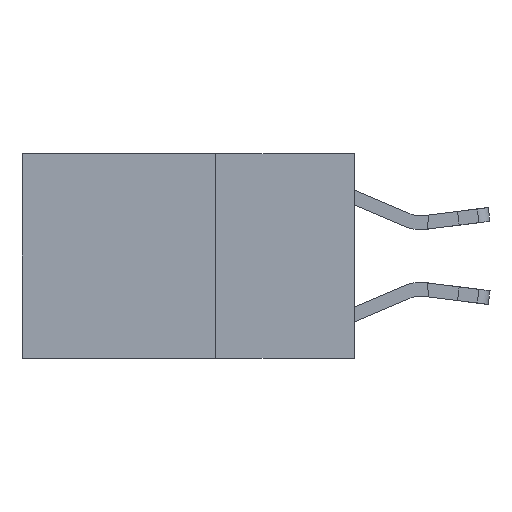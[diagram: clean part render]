
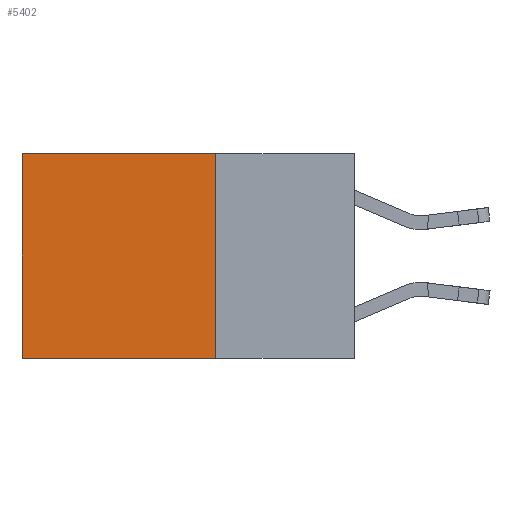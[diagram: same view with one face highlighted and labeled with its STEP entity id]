
A CAD part, left-side view. The second image highlights one B-rep face of the part: STEP entity #5402.
In plain terms, the highlighted planar face has unit normal (-1, 0, 0).
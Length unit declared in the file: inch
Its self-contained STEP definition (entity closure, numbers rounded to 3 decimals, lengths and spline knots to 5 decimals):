
#186 = VERTEX_POINT ( 'NONE', #7719 ) ;
#538 = FACE_OUTER_BOUND ( 'NONE', #6070, .T. ) ;
#646 = CARTESIAN_POINT ( 'NONE',  ( 0.2625, 0.25, -0.37 ) ) ;
#1279 = DIRECTION ( 'NONE',  ( 0., 0., -1. ) ) ;
#1667 = ORIENTED_EDGE ( 'NONE', *, *, #12426, .T. ) ;
#1737 = VECTOR ( 'NONE', #9264, 39.37008 ) ;
#2092 = LINE ( 'NONE', #6153, #11781 ) ;
#2173 = CARTESIAN_POINT ( 'NONE',  ( 0.2625, 0.25, -0.37 ) ) ;
#3585 = PLANE ( 'NONE',  #8578 ) ;
#4514 = EDGE_CURVE ( 'NONE', #4970, #6692, #2092, .T. ) ;
#4708 = CARTESIAN_POINT ( 'NONE',  ( 0.2625, 0.25, 0. ) ) ;
#4970 = VERTEX_POINT ( 'NONE', #4708 ) ;
#5058 = ORIENTED_EDGE ( 'NONE', *, *, #4514, .F. ) ;
#5220 = VERTEX_POINT ( 'NONE', #9020 ) ;
#5402 = ADVANCED_FACE ( 'NONE', ( #538 ), #3585, .F. ) ;
#5512 = DIRECTION ( 'NONE',  ( 0., 0., -1. ) ) ;
#6070 = EDGE_LOOP ( 'NONE', ( #10207, #8852, #5058, #1667 ) ) ;
#6153 = CARTESIAN_POINT ( 'NONE',  ( 0.2625, 0.25, 0. ) ) ;
#6442 = VECTOR ( 'NONE', #8548, 39.37008 ) ;
#6692 = VERTEX_POINT ( 'NONE', #2173 ) ;
#7056 = LINE ( 'NONE', #646, #6442 ) ;
#7464 = VECTOR ( 'NONE', #1279, 39.37008 ) ;
#7719 = CARTESIAN_POINT ( 'NONE',  ( 0.2625, 0.6, 0. ) ) ;
#8091 = CARTESIAN_POINT ( 'NONE',  ( 0.2625, 0.6, 0. ) ) ;
#8204 = EDGE_CURVE ( 'NONE', #186, #5220, #10079, .T. ) ;
#8242 = CARTESIAN_POINT ( 'NONE',  ( 0.2625, 0.25, 0. ) ) ;
#8548 = DIRECTION ( 'NONE',  ( 0., 1., 0. ) ) ;
#8578 = AXIS2_PLACEMENT_3D ( 'NONE', #10422, #11346, #5512 ) ;
#8852 = ORIENTED_EDGE ( 'NONE', *, *, #12684, .F. ) ;
#9020 = CARTESIAN_POINT ( 'NONE',  ( 0.2625, 0.6, -0.37 ) ) ;
#9210 = LINE ( 'NONE', #8242, #1737 ) ;
#9264 = DIRECTION ( 'NONE',  ( 0., 1., 0. ) ) ;
#10079 = LINE ( 'NONE', #8091, #7464 ) ;
#10207 = ORIENTED_EDGE ( 'NONE', *, *, #8204, .T. ) ;
#10422 = CARTESIAN_POINT ( 'NONE',  ( 0.2625, 0.25, 0. ) ) ;
#11346 = DIRECTION ( 'NONE',  ( 1., 0., 0. ) ) ;
#11781 = VECTOR ( 'NONE', #11973, 39.37008 ) ;
#11973 = DIRECTION ( 'NONE',  ( 0., 0., -1. ) ) ;
#12426 = EDGE_CURVE ( 'NONE', #4970, #186, #9210, .T. ) ;
#12684 = EDGE_CURVE ( 'NONE', #6692, #5220, #7056, .T. ) ;
